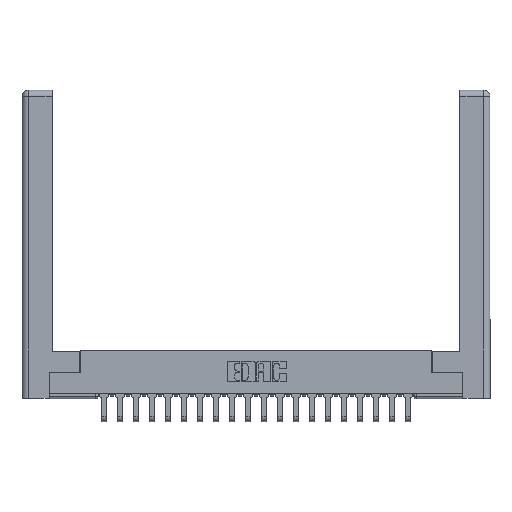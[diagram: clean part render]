
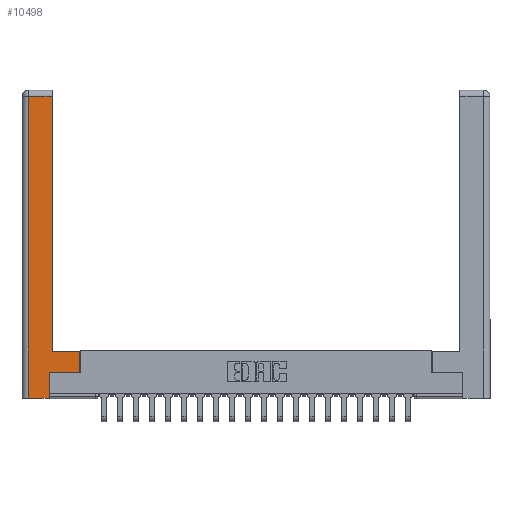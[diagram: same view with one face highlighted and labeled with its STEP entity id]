
A CAD part, top view. The second image highlights one B-rep face of the part: STEP entity #10498.
In plain terms, the highlighted planar face has unit normal (0, 0, 1).
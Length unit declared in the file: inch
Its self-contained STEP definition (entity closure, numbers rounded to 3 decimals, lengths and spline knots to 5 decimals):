
#703 = LINE ( 'NONE', #15895, #11922 ) ;
#1643 = VECTOR ( 'NONE', #2657, 39.37008 ) ;
#2409 = CARTESIAN_POINT ( 'NONE',  ( 0.265, 0., 0. ) ) ;
#2657 = DIRECTION ( 'NONE',  ( 1., 0., 0. ) ) ;
#2843 = LINE ( 'NONE', #22228, #24602 ) ;
#3286 = ORIENTED_EDGE ( 'NONE', *, *, #18747, .T. ) ;
#3861 = DIRECTION ( 'NONE',  ( -1., 0., 0. ) ) ;
#4156 = ORIENTED_EDGE ( 'NONE', *, *, #22748, .T. ) ;
#4426 = EDGE_CURVE ( 'NONE', #5291, #15619, #2843, .T. ) ;
#4619 = AXIS2_PLACEMENT_3D ( 'NONE', #13440, #15074, #3861 ) ;
#5291 = VERTEX_POINT ( 'NONE', #12074 ) ;
#5438 = ORIENTED_EDGE ( 'NONE', *, *, #6971, .T. ) ;
#5702 = VERTEX_POINT ( 'NONE', #12057 ) ;
#6291 = DIRECTION ( 'NONE',  ( 1., 0., 0. ) ) ;
#6692 = DIRECTION ( 'NONE',  ( -1., 0., 0. ) ) ;
#6803 = DIRECTION ( 'NONE',  ( 0., 1., 0. ) ) ;
#6925 = CARTESIAN_POINT ( 'NONE',  ( 0.0615, 2.94, 0. ) ) ;
#6971 = EDGE_CURVE ( 'NONE', #13926, #14314, #10669, .T. ) ;
#7063 = EDGE_LOOP ( 'NONE', ( #23568, #18775, #23711, #4156, #24173, #15744, #5438, #3286 ) ) ;
#7589 = VECTOR ( 'NONE', #8079, 39.37008 ) ;
#8079 = DIRECTION ( 'NONE',  ( 0., 1., 0. ) ) ;
#8515 = EDGE_CURVE ( 'NONE', #10734, #13926, #16084, .T. ) ;
#8675 = CARTESIAN_POINT ( 'NONE',  ( 0.565, 0.45, 0. ) ) ;
#8803 = CARTESIAN_POINT ( 'NONE',  ( 0.0615, 0., 0. ) ) ;
#9094 = VECTOR ( 'NONE', #6803, 39.37008 ) ;
#9278 = DIRECTION ( 'NONE',  ( 0., -1., 0. ) ) ;
#10094 = CARTESIAN_POINT ( 'NONE',  ( 0.265, 0.245, 0. ) ) ;
#10498 = ADVANCED_FACE ( 'NONE', ( #22517 ), #20890, .F. ) ;
#10669 = LINE ( 'NONE', #8675, #9094 ) ;
#10670 = LINE ( 'NONE', #8803, #17572 ) ;
#10734 = VERTEX_POINT ( 'NONE', #10094 ) ;
#11230 = CARTESIAN_POINT ( 'NONE',  ( 0.565, 0.245, 0. ) ) ;
#11588 = EDGE_CURVE ( 'NONE', #15619, #21945, #16249, .T. ) ;
#11711 = VECTOR ( 'NONE', #6291, 39.37008 ) ;
#11762 = CARTESIAN_POINT ( 'NONE',  ( 0.565, 0.245, 0. ) ) ;
#11922 = VECTOR ( 'NONE', #23488, 39.37008 ) ;
#12057 = CARTESIAN_POINT ( 'NONE',  ( 0.265, 0., 0. ) ) ;
#12074 = CARTESIAN_POINT ( 'NONE',  ( 0.295, 0.45, 0. ) ) ;
#12771 = CARTESIAN_POINT ( 'NONE',  ( 0.295, 2.94, 0. ) ) ;
#13440 = CARTESIAN_POINT ( 'NONE',  ( 0., 0., 0. ) ) ;
#13926 = VERTEX_POINT ( 'NONE', #11230 ) ;
#14314 = VERTEX_POINT ( 'NONE', #16884 ) ;
#15074 = DIRECTION ( 'NONE',  ( 0., 0., -1. ) ) ;
#15619 = VERTEX_POINT ( 'NONE', #12771 ) ;
#15744 = ORIENTED_EDGE ( 'NONE', *, *, #8515, .T. ) ;
#15760 = VECTOR ( 'NONE', #6692, 39.37008 ) ;
#15895 = CARTESIAN_POINT ( 'NONE',  ( 0.295, 0.45, 0. ) ) ;
#16084 = LINE ( 'NONE', #11762, #11711 ) ;
#16249 = LINE ( 'NONE', #6925, #15760 ) ;
#16381 = DIRECTION ( 'NONE',  ( 0., 1., 0. ) ) ;
#16884 = CARTESIAN_POINT ( 'NONE',  ( 0.565, 0.45, 0. ) ) ;
#17572 = VECTOR ( 'NONE', #9278, 39.37008 ) ;
#18747 = EDGE_CURVE ( 'NONE', #14314, #5291, #703, .T. ) ;
#18775 = ORIENTED_EDGE ( 'NONE', *, *, #11588, .T. ) ;
#19386 = LINE ( 'NONE', #23610, #7589 ) ;
#19569 = LINE ( 'NONE', #2409, #1643 ) ;
#20890 = PLANE ( 'NONE',  #4619 ) ;
#21486 = CARTESIAN_POINT ( 'NONE',  ( 0.0615, 2.94, 0. ) ) ;
#21791 = CARTESIAN_POINT ( 'NONE',  ( 0.0615, 0., 0. ) ) ;
#21869 = EDGE_CURVE ( 'NONE', #5702, #10734, #19386, .T. ) ;
#21945 = VERTEX_POINT ( 'NONE', #21486 ) ;
#22228 = CARTESIAN_POINT ( 'NONE',  ( 0.295, 3., 0. ) ) ;
#22517 = FACE_OUTER_BOUND ( 'NONE', #7063, .T. ) ;
#22748 = EDGE_CURVE ( 'NONE', #22899, #5702, #19569, .T. ) ;
#22899 = VERTEX_POINT ( 'NONE', #21791 ) ;
#23488 = DIRECTION ( 'NONE',  ( -1., 0., 0. ) ) ;
#23568 = ORIENTED_EDGE ( 'NONE', *, *, #4426, .T. ) ;
#23605 = EDGE_CURVE ( 'NONE', #21945, #22899, #10670, .T. ) ;
#23610 = CARTESIAN_POINT ( 'NONE',  ( 0.265, 0.245, 0. ) ) ;
#23711 = ORIENTED_EDGE ( 'NONE', *, *, #23605, .T. ) ;
#24173 = ORIENTED_EDGE ( 'NONE', *, *, #21869, .T. ) ;
#24602 = VECTOR ( 'NONE', #16381, 39.37008 ) ;
